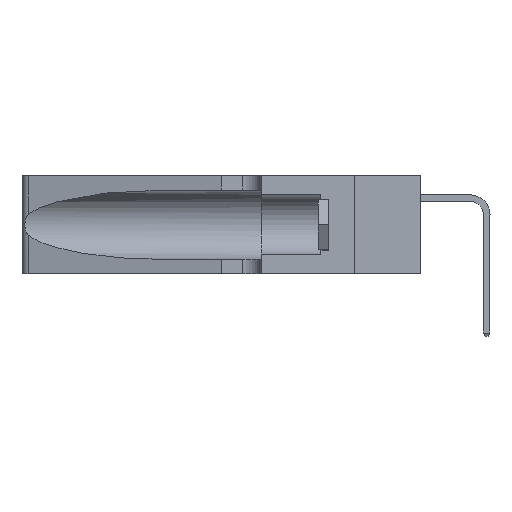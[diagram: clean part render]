
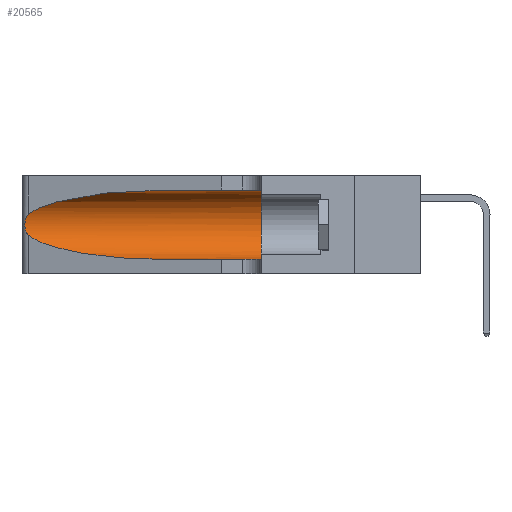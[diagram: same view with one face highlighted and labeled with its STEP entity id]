
A CAD part, left-side view. The second image highlights one B-rep face of the part: STEP entity #20565.
In plain terms, the highlighted cylindrical face has radius 3.308 mm (diameter 6.617 mm), a partial arc.
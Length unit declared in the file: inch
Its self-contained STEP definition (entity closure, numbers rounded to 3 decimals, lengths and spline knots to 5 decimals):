
#207 =( BOUNDED_CURVE ( )  B_SPLINE_CURVE ( 3, ( #2590, #16851, #5024, #21622 ),
 .UNSPECIFIED., .F., .T. ) 
 B_SPLINE_CURVE_WITH_KNOTS ( ( 4, 4 ),
 ( 3.44316, 4.71239 ),
 .UNSPECIFIED. ) 
 CURVE ( )  GEOMETRIC_REPRESENTATION_ITEM ( )  RATIONAL_B_SPLINE_CURVE ( ( 1., 0.87, 0.87, 1. ) ) 
 REPRESENTATION_ITEM ( '' )  );
#1956 = ORIENTED_EDGE ( 'NONE', *, *, #11686, .T. ) ;
#2267 = CARTESIAN_POINT ( 'NONE',  ( 0.25787, 1.23484, 0.2124 ) ) ;
#2338 = CARTESIAN_POINT ( 'NONE',  ( 0.2373, 1.15595, 0.28018 ) ) ;
#2590 = CARTESIAN_POINT ( 'NONE',  ( 0.25487, 1.22718, 0.14631 ) ) ;
#2772 = ORIENTED_EDGE ( 'NONE', *, *, #15483, .T. ) ;
#3268 = ORIENTED_EDGE ( 'NONE', *, *, #25965, .F. ) ;
#3698 = AXIS2_PLACEMENT_3D ( 'NONE', #8952, #25500, #11327 ) ;
#3789 = DIRECTION ( 'NONE',  ( 0., -1., 0. ) ) ;
#4702 = CARTESIAN_POINT ( 'NONE',  ( 0.26018, 1.23835, 0.19895 ) ) ;
#4777 = CARTESIAN_POINT ( 'NONE',  ( 0.18966, 0.96281, 0.31525 ) ) ;
#5024 = CARTESIAN_POINT ( 'NONE',  ( 0.18966, 0.96281, 0.05475 ) ) ;
#5056 = VERTEX_POINT ( 'NONE', #21837 ) ;
#5235 = ORIENTED_EDGE ( 'NONE', *, *, #6969, .T. ) ;
#5358 = CIRCLE ( 'NONE', #3698, 0.13025 ) ;
#5587 = DIRECTION ( 'NONE',  ( 0., 0., -1. ) ) ;
#6188 = CARTESIAN_POINT ( 'NONE',  ( 0.1305, 1.61858, 0.31525 ) ) ;
#6236 = VECTOR ( 'NONE', #3789, 39.37008 ) ;
#6284 = EDGE_LOOP ( 'NONE', ( #5235, #1956, #17536, #2772, #3268, #13974 ) ) ;
#6969 = EDGE_CURVE ( 'NONE', #19759, #27161, #30520, .T. ) ;
#7112 = CARTESIAN_POINT ( 'NONE',  ( 0.26075, 1.23896, 0.178 ) ) ;
#8952 = CARTESIAN_POINT ( 'NONE',  ( 0.1305, 0.35, 0.185 ) ) ;
#9410 = CARTESIAN_POINT ( 'NONE',  ( 0.25555, 1.22994, 0.2215 ) ) ;
#9498 = CARTESIAN_POINT ( 'NONE',  ( 0.25856, 1.23593, 0.16098 ) ) ;
#9580 = CARTESIAN_POINT ( 'NONE',  ( 0.25487, 1.22718, 0.22369 ) ) ;
#10812 = VERTEX_POINT ( 'NONE', #15006 ) ;
#11327 = DIRECTION ( 'NONE',  ( 0., 0., 1. ) ) ;
#11546 = CYLINDRICAL_SURFACE ( 'NONE', #21280, 0.13025 ) ;
#11686 = EDGE_CURVE ( 'NONE', #27161, #15908, #23754, .T. ) ;
#11863 = CARTESIAN_POINT ( 'NONE',  ( 0.25639, 1.23186, 0.15144 ) ) ;
#12728 = DIRECTION ( 'NONE',  ( 0., -1., 0. ) ) ;
#13395 = VECTOR ( 'NONE', #27849, 39.37008 ) ;
#13974 = ORIENTED_EDGE ( 'NONE', *, *, #15987, .F. ) ;
#14232 = CARTESIAN_POINT ( 'NONE',  ( 0.25487, 1.22718, 0.14631 ) ) ;
#15006 = CARTESIAN_POINT ( 'NONE',  ( 0.1305, 0.72297, 0.05475 ) ) ;
#15483 = EDGE_CURVE ( 'NONE', #10812, #24900, #20443, .T. ) ;
#15908 = VERTEX_POINT ( 'NONE', #24862 ) ;
#15987 = EDGE_CURVE ( 'NONE', #19759, #5056, #18832, .T. ) ;
#16243 = CARTESIAN_POINT ( 'NONE',  ( 0.1305, 0.35, 0.05475 ) ) ;
#16523 = CARTESIAN_POINT ( 'NONE',  ( 0.25639, 1.23184, 0.21858 ) ) ;
#16851 = CARTESIAN_POINT ( 'NONE',  ( 0.2373, 1.15595, 0.08982 ) ) ;
#17536 = ORIENTED_EDGE ( 'NONE', *, *, #19226, .T. ) ;
#18575 = FACE_OUTER_BOUND ( 'NONE', #6284, .T. ) ;
#18832 = LINE ( 'NONE', #6188, #6236 ) ;
#18901 = CARTESIAN_POINT ( 'NONE',  ( 0.25854, 1.2359, 0.20912 ) ) ;
#19226 = EDGE_CURVE ( 'NONE', #15908, #10812, #207, .T. ) ;
#19759 = VERTEX_POINT ( 'NONE', #20961 ) ;
#20443 = LINE ( 'NONE', #30214, #13395 ) ;
#20565 = ADVANCED_FACE ( 'NONE', ( #18575 ), #11546, .F. ) ;
#20961 = CARTESIAN_POINT ( 'NONE',  ( 0.1305, 0.72297, 0.31525 ) ) ;
#21280 = AXIS2_PLACEMENT_3D ( 'NONE', #24568, #12728, #5587 ) ;
#21295 = CARTESIAN_POINT ( 'NONE',  ( 0.26075, 1.23896, 0.19203 ) ) ;
#21622 = CARTESIAN_POINT ( 'NONE',  ( 0.1305, 0.72297, 0.05475 ) ) ;
#21837 = CARTESIAN_POINT ( 'NONE',  ( 0.1305, 0.35, 0.31525 ) ) ;
#23682 = CARTESIAN_POINT ( 'NONE',  ( 0.26017, 1.23833, 0.17102 ) ) ;
#23754 = B_SPLINE_CURVE_WITH_KNOTS ( 'NONE', 3,
 ( #25951, #9410, #16523, #2267, #18901, #4702, #21295, #7112, #23682, #9498, #26054, #11863, #28413, #14232 ),
 .UNSPECIFIED., .F., .F.,
 ( 4, 2, 2, 2, 2, 2, 4 ),
 ( 0., 0.00027, 0.00053, 0.00107, 0.0016, 0.00187, 0.00214 ),
 .UNSPECIFIED. ) ;
#23766 = CARTESIAN_POINT ( 'NONE',  ( 0.1305, 0.72297, 0.31525 ) ) ;
#24568 = CARTESIAN_POINT ( 'NONE',  ( 0.1305, 1.61858, 0.185 ) ) ;
#24862 = CARTESIAN_POINT ( 'NONE',  ( 0.25487, 1.22718, 0.14631 ) ) ;
#24900 = VERTEX_POINT ( 'NONE', #16243 ) ;
#25500 = DIRECTION ( 'NONE',  ( 0., 1., 0. ) ) ;
#25951 = CARTESIAN_POINT ( 'NONE',  ( 0.25487, 1.22718, 0.22369 ) ) ;
#25965 = EDGE_CURVE ( 'NONE', #5056, #24900, #5358, .T. ) ;
#26054 = CARTESIAN_POINT ( 'NONE',  ( 0.25789, 1.23486, 0.15765 ) ) ;
#27161 = VERTEX_POINT ( 'NONE', #27795 ) ;
#27795 = CARTESIAN_POINT ( 'NONE',  ( 0.25487, 1.22718, 0.22369 ) ) ;
#27849 = DIRECTION ( 'NONE',  ( 0., -1., 0. ) ) ;
#28413 = CARTESIAN_POINT ( 'NONE',  ( 0.25555, 1.22993, 0.14849 ) ) ;
#30214 = CARTESIAN_POINT ( 'NONE',  ( 0.1305, 1.61858, 0.05475 ) ) ;
#30520 =( BOUNDED_CURVE ( )  B_SPLINE_CURVE ( 3, ( #23766, #4777, #2338, #9580 ),
 .UNSPECIFIED., .F., .T. ) 
 B_SPLINE_CURVE_WITH_KNOTS ( ( 4, 4 ),
 ( 1.5708, 2.84003 ),
 .UNSPECIFIED. ) 
 CURVE ( )  GEOMETRIC_REPRESENTATION_ITEM ( )  RATIONAL_B_SPLINE_CURVE ( ( 1., 0.87, 0.87, 1. ) ) 
 REPRESENTATION_ITEM ( '' )  );
